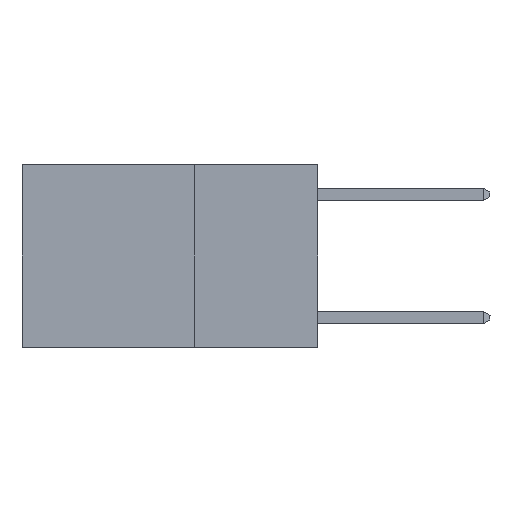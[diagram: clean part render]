
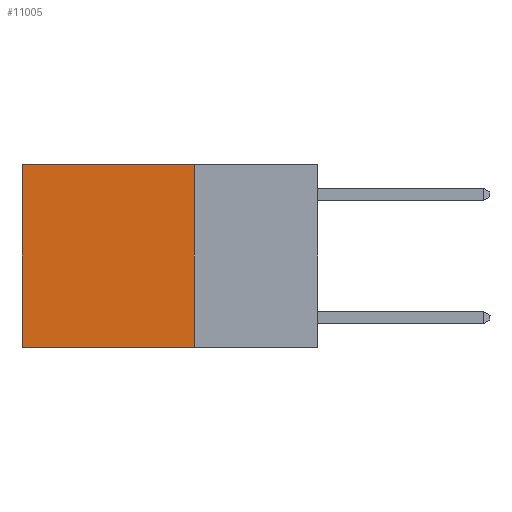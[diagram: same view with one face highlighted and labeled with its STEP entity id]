
A CAD part, left-side view. The second image highlights one B-rep face of the part: STEP entity #11005.
In plain terms, the highlighted planar face has unit normal (-1, 0, 0).
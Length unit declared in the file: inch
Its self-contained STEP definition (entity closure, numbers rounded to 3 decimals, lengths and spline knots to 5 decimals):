
#13 = VECTOR ( 'NONE', #8166, 39.37008 ) ;
#675 = DIRECTION ( 'NONE',  ( 0., 0., -1. ) ) ;
#1173 = ORIENTED_EDGE ( 'NONE', *, *, #9097, .F. ) ;
#1698 = DIRECTION ( 'NONE',  ( 1., 0., 0. ) ) ;
#2734 = CARTESIAN_POINT ( 'NONE',  ( 0.2625, 0.25, -0.37 ) ) ;
#3005 = VERTEX_POINT ( 'NONE', #10977 ) ;
#3044 = LINE ( 'NONE', #4186, #10045 ) ;
#4186 = CARTESIAN_POINT ( 'NONE',  ( 0.2625, 0.25, 0. ) ) ;
#4338 = AXIS2_PLACEMENT_3D ( 'NONE', #5698, #1698, #675 ) ;
#4774 = ORIENTED_EDGE ( 'NONE', *, *, #11825, .T. ) ;
#5665 = CARTESIAN_POINT ( 'NONE',  ( 0.2625, 0.6, 0. ) ) ;
#5698 = CARTESIAN_POINT ( 'NONE',  ( 0.2625, 0.25, 0. ) ) ;
#5922 = ORIENTED_EDGE ( 'NONE', *, *, #6015, .T. ) ;
#6015 = EDGE_CURVE ( 'NONE', #11128, #3005, #12488, .T. ) ;
#6213 = DIRECTION ( 'NONE',  ( 0., 0., -1. ) ) ;
#6733 = PLANE ( 'NONE',  #4338 ) ;
#6942 = VECTOR ( 'NONE', #6213, 39.37008 ) ;
#7070 = VERTEX_POINT ( 'NONE', #11153 ) ;
#7542 = DIRECTION ( 'NONE',  ( 0., 1., 0. ) ) ;
#8166 = DIRECTION ( 'NONE',  ( 0., 1., 0. ) ) ;
#8377 = EDGE_LOOP ( 'NONE', ( #5922, #13045, #1173, #4774 ) ) ;
#9097 = EDGE_CURVE ( 'NONE', #7070, #12147, #9299, .T. ) ;
#9299 = LINE ( 'NONE', #13542, #6942 ) ;
#9742 = FACE_OUTER_BOUND ( 'NONE', #8377, .T. ) ;
#9746 = DIRECTION ( 'NONE',  ( 0., 0., -1. ) ) ;
#9881 = CARTESIAN_POINT ( 'NONE',  ( 0.2625, 0.6, 0. ) ) ;
#10045 = VECTOR ( 'NONE', #7542, 39.37008 ) ;
#10977 = CARTESIAN_POINT ( 'NONE',  ( 0.2625, 0.6, -0.37 ) ) ;
#11005 = ADVANCED_FACE ( 'NONE', ( #9742 ), #6733, .F. ) ;
#11128 = VERTEX_POINT ( 'NONE', #5665 ) ;
#11153 = CARTESIAN_POINT ( 'NONE',  ( 0.2625, 0.25, 0. ) ) ;
#11340 = EDGE_CURVE ( 'NONE', #12147, #3005, #12187, .T. ) ;
#11825 = EDGE_CURVE ( 'NONE', #7070, #11128, #3044, .T. ) ;
#12147 = VERTEX_POINT ( 'NONE', #2734 ) ;
#12187 = LINE ( 'NONE', #13158, #13 ) ;
#12334 = VECTOR ( 'NONE', #9746, 39.37008 ) ;
#12488 = LINE ( 'NONE', #9881, #12334 ) ;
#13045 = ORIENTED_EDGE ( 'NONE', *, *, #11340, .F. ) ;
#13158 = CARTESIAN_POINT ( 'NONE',  ( 0.2625, 0.25, -0.37 ) ) ;
#13542 = CARTESIAN_POINT ( 'NONE',  ( 0.2625, 0.25, 0. ) ) ;
